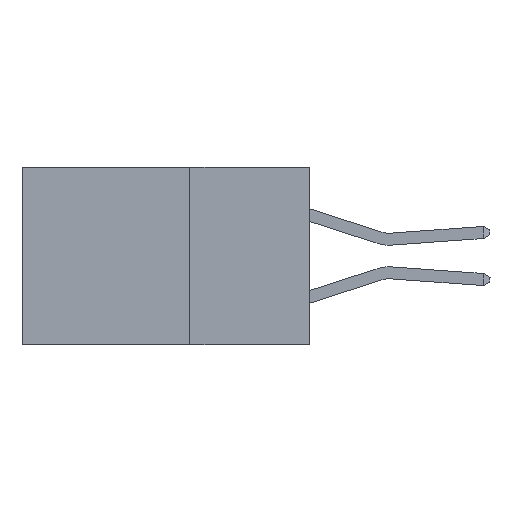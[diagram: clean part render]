
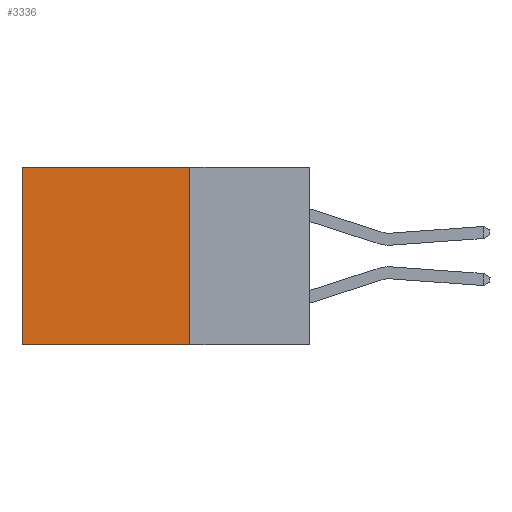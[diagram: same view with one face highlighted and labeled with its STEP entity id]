
A CAD part, left-side view. The second image highlights one B-rep face of the part: STEP entity #3336.
In plain terms, the highlighted planar face has unit normal (-1, 0, 0).
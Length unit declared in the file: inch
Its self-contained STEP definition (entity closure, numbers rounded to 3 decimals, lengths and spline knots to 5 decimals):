
#486 = LINE ( 'NONE', #12270, #6683 ) ;
#574 = CARTESIAN_POINT ( 'NONE',  ( 0.298, 0.6, 0. ) ) ;
#952 = ORIENTED_EDGE ( 'NONE', *, *, #5987, .T. ) ;
#987 = LINE ( 'NONE', #11703, #6068 ) ;
#1172 = EDGE_CURVE ( 'NONE', #7121, #13136, #10916, .T. ) ;
#1983 = DIRECTION ( 'NONE',  ( 0., 0., -1. ) ) ;
#2283 = CARTESIAN_POINT ( 'NONE',  ( 0.298, 0.25, 0. ) ) ;
#3165 = DIRECTION ( 'NONE',  ( 0., 0., -1. ) ) ;
#3301 = DIRECTION ( 'NONE',  ( 1., 0., 0. ) ) ;
#3336 = ADVANCED_FACE ( 'NONE', ( #6234 ), #12429, .F. ) ;
#3673 = CARTESIAN_POINT ( 'NONE',  ( 0.298, 0.25, -0.37 ) ) ;
#5692 = ORIENTED_EDGE ( 'NONE', *, *, #7103, .F. ) ;
#5987 = EDGE_CURVE ( 'NONE', #8322, #12153, #486, .T. ) ;
#6068 = VECTOR ( 'NONE', #6660, 39.37008 ) ;
#6234 = FACE_OUTER_BOUND ( 'NONE', #10281, .T. ) ;
#6660 = DIRECTION ( 'NONE',  ( 0., 0., -1. ) ) ;
#6683 = VECTOR ( 'NONE', #12224, 39.37008 ) ;
#6909 = VECTOR ( 'NONE', #12715, 39.37008 ) ;
#7103 = EDGE_CURVE ( 'NONE', #8322, #7121, #8100, .T. ) ;
#7121 = VERTEX_POINT ( 'NONE', #11347 ) ;
#8100 = LINE ( 'NONE', #8157, #12255 ) ;
#8157 = CARTESIAN_POINT ( 'NONE',  ( 0.298, 0.25, 0. ) ) ;
#8322 = VERTEX_POINT ( 'NONE', #11612 ) ;
#8415 = ORIENTED_EDGE ( 'NONE', *, *, #1172, .F. ) ;
#9364 = CARTESIAN_POINT ( 'NONE',  ( 0.298, 0.6, -0.37 ) ) ;
#10281 = EDGE_LOOP ( 'NONE', ( #12981, #8415, #5692, #952 ) ) ;
#10916 = LINE ( 'NONE', #3673, #6909 ) ;
#11347 = CARTESIAN_POINT ( 'NONE',  ( 0.298, 0.25, -0.37 ) ) ;
#11612 = CARTESIAN_POINT ( 'NONE',  ( 0.298, 0.25, 0. ) ) ;
#11699 = AXIS2_PLACEMENT_3D ( 'NONE', #2283, #3301, #3165 ) ;
#11703 = CARTESIAN_POINT ( 'NONE',  ( 0.298, 0.6, 0. ) ) ;
#12153 = VERTEX_POINT ( 'NONE', #574 ) ;
#12160 = EDGE_CURVE ( 'NONE', #12153, #13136, #987, .T. ) ;
#12224 = DIRECTION ( 'NONE',  ( 0., 1., 0. ) ) ;
#12255 = VECTOR ( 'NONE', #1983, 39.37008 ) ;
#12270 = CARTESIAN_POINT ( 'NONE',  ( 0.298, 0.25, 0. ) ) ;
#12429 = PLANE ( 'NONE',  #11699 ) ;
#12715 = DIRECTION ( 'NONE',  ( 0., 1., 0. ) ) ;
#12981 = ORIENTED_EDGE ( 'NONE', *, *, #12160, .T. ) ;
#13136 = VERTEX_POINT ( 'NONE', #9364 ) ;
